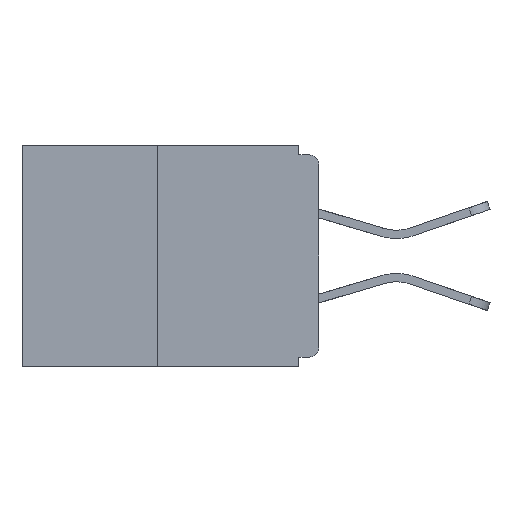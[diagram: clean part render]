
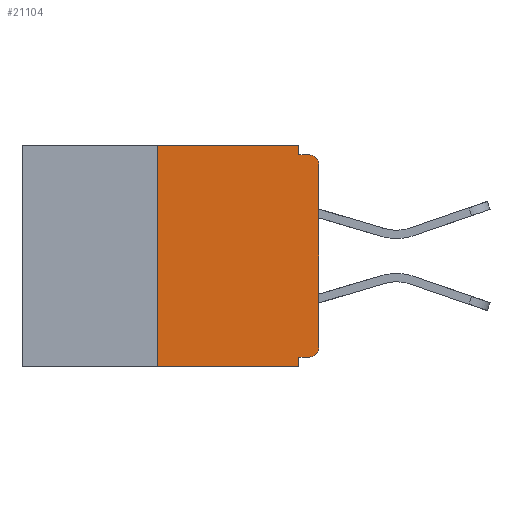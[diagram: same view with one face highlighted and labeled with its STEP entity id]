
A CAD part, left-side view. The second image highlights one B-rep face of the part: STEP entity #21104.
In plain terms, the highlighted planar face has unit normal (-1, 0, 0).
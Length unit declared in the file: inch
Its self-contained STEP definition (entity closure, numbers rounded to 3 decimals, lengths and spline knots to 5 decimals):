
#476 = DIRECTION ( 'NONE',  ( 0., 0., 1. ) ) ;
#1925 = ORIENTED_EDGE ( 'NONE', *, *, #23417, .F. ) ;
#2203 = VERTEX_POINT ( 'NONE', #7121 ) ;
#2289 = EDGE_CURVE ( 'NONE', #20654, #20920, #18518, .T. ) ;
#2533 = CARTESIAN_POINT ( 'NONE',  ( 0., 0.46, 0. ) ) ;
#2601 = EDGE_LOOP ( 'NONE', ( #22878, #6799, #9695, #23954, #12392, #19267, #4826, #17020, #1925, #10896 ) ) ;
#2767 = PLANE ( 'NONE',  #15764 ) ;
#2770 = CARTESIAN_POINT ( 'NONE',  ( 0., 0.25, 0. ) ) ;
#3852 = EDGE_CURVE ( 'NONE', #21690, #20055, #19896, .T. ) ;
#4244 = CARTESIAN_POINT ( 'NONE',  ( 0., 0.46, 0. ) ) ;
#4379 = VERTEX_POINT ( 'NONE', #20947 ) ;
#4826 = ORIENTED_EDGE ( 'NONE', *, *, #19658, .T. ) ;
#5192 = FACE_OUTER_BOUND ( 'NONE', #2601, .T. ) ;
#5286 = EDGE_CURVE ( 'NONE', #2203, #10711, #18366, .T. ) ;
#5598 = VERTEX_POINT ( 'NONE', #2770 ) ;
#5928 = VECTOR ( 'NONE', #20746, 39.37008 ) ;
#5968 = LINE ( 'NONE', #9209, #15302 ) ;
#6614 = VECTOR ( 'NONE', #17550, 39.37008 ) ;
#6799 = ORIENTED_EDGE ( 'NONE', *, *, #11990, .F. ) ;
#6907 = DIRECTION ( 'NONE',  ( 0., 0., -1. ) ) ;
#7121 = CARTESIAN_POINT ( 'NONE',  ( 0., 0.015, -0.328 ) ) ;
#7600 = DIRECTION ( 'NONE',  ( 0., 0., 1. ) ) ;
#7608 = DIRECTION ( 'NONE',  ( 0., 0., -1. ) ) ;
#7789 = EDGE_CURVE ( 'NONE', #2203, #23434, #19335, .T. ) ;
#7893 = VECTOR ( 'NONE', #19239, 39.37008 ) ;
#8104 = LINE ( 'NONE', #13598, #12831 ) ;
#9209 = CARTESIAN_POINT ( 'NONE',  ( 0., 0.031, 0. ) ) ;
#9425 = CARTESIAN_POINT ( 'NONE',  ( 0., 0., -0.015 ) ) ;
#9695 = ORIENTED_EDGE ( 'NONE', *, *, #3852, .T. ) ;
#9781 = VECTOR ( 'NONE', #24163, 39.37008 ) ;
#10086 = DIRECTION ( 'NONE',  ( 1., 0., 0. ) ) ;
#10711 = VERTEX_POINT ( 'NONE', #21001 ) ;
#10741 = EDGE_CURVE ( 'NONE', #5598, #19440, #15689, .T. ) ;
#10896 = ORIENTED_EDGE ( 'NONE', *, *, #11846, .F. ) ;
#11138 = CARTESIAN_POINT ( 'NONE',  ( 0., 0.031, 0. ) ) ;
#11846 = EDGE_CURVE ( 'NONE', #19440, #4379, #5968, .T. ) ;
#11990 = EDGE_CURVE ( 'NONE', #21690, #5598, #22936, .T. ) ;
#12392 = ORIENTED_EDGE ( 'NONE', *, *, #7789, .F. ) ;
#12660 = CARTESIAN_POINT ( 'NONE',  ( 0., 0., -0.03 ) ) ;
#12831 = VECTOR ( 'NONE', #476, 39.37008 ) ;
#13597 = LINE ( 'NONE', #14649, #9781 ) ;
#13598 = CARTESIAN_POINT ( 'NONE',  ( 0., 0., 0. ) ) ;
#14649 = CARTESIAN_POINT ( 'NONE',  ( 0., 0.031, -0.343 ) ) ;
#14977 = CARTESIAN_POINT ( 'NONE',  ( 0., 0.031, -0.328 ) ) ;
#15013 = CARTESIAN_POINT ( 'NONE',  ( 0., 0.25, 0. ) ) ;
#15017 = DIRECTION ( 'NONE',  ( -1., 0., 0. ) ) ;
#15302 = VECTOR ( 'NONE', #16848, 39.37008 ) ;
#15539 = CARTESIAN_POINT ( 'NONE',  ( 0., 0.46, -0.343 ) ) ;
#15664 = AXIS2_PLACEMENT_3D ( 'NONE', #17167, #15017, #7608 ) ;
#15689 = LINE ( 'NONE', #4244, #6614 ) ;
#15764 = AXIS2_PLACEMENT_3D ( 'NONE', #2533, #10086, #23194 ) ;
#16848 = DIRECTION ( 'NONE',  ( 0., 0., -1. ) ) ;
#17020 = ORIENTED_EDGE ( 'NONE', *, *, #2289, .T. ) ;
#17054 = LINE ( 'NONE', #9425, #5928 ) ;
#17167 = CARTESIAN_POINT ( 'NONE',  ( 0., 0.015, -0.03 ) ) ;
#17550 = DIRECTION ( 'NONE',  ( 0., -1., 0. ) ) ;
#17764 = CARTESIAN_POINT ( 'NONE',  ( 0., 0.25, -0.343 ) ) ;
#17944 = CARTESIAN_POINT ( 'NONE',  ( 0., 0.015, -0.313 ) ) ;
#17952 = VECTOR ( 'NONE', #7600, 39.37008 ) ;
#18366 = CIRCLE ( 'NONE', #20612, 0.015 ) ;
#18442 = VECTOR ( 'NONE', #23558, 39.37008 ) ;
#18518 = CIRCLE ( 'NONE', #15664, 0.015 ) ;
#19239 = DIRECTION ( 'NONE',  ( 0., -1., 0. ) ) ;
#19267 = ORIENTED_EDGE ( 'NONE', *, *, #5286, .T. ) ;
#19335 = LINE ( 'NONE', #21671, #18442 ) ;
#19440 = VERTEX_POINT ( 'NONE', #11138 ) ;
#19658 = EDGE_CURVE ( 'NONE', #10711, #20654, #8104, .T. ) ;
#19896 = LINE ( 'NONE', #15539, #7893 ) ;
#19999 = DIRECTION ( 'NONE',  ( -1., 0., 0. ) ) ;
#20055 = VERTEX_POINT ( 'NONE', #20285 ) ;
#20285 = CARTESIAN_POINT ( 'NONE',  ( 0., 0.031, -0.343 ) ) ;
#20612 = AXIS2_PLACEMENT_3D ( 'NONE', #17944, #19999, #6907 ) ;
#20654 = VERTEX_POINT ( 'NONE', #12660 ) ;
#20746 = DIRECTION ( 'NONE',  ( 0., -1., 0. ) ) ;
#20920 = VERTEX_POINT ( 'NONE', #22708 ) ;
#20947 = CARTESIAN_POINT ( 'NONE',  ( 0., 0.031, -0.015 ) ) ;
#21001 = CARTESIAN_POINT ( 'NONE',  ( 0., 0., -0.313 ) ) ;
#21104 = ADVANCED_FACE ( 'NONE', ( #5192 ), #2767, .F. ) ;
#21671 = CARTESIAN_POINT ( 'NONE',  ( 0., 0., -0.328 ) ) ;
#21690 = VERTEX_POINT ( 'NONE', #17764 ) ;
#22033 = EDGE_CURVE ( 'NONE', #23434, #20055, #13597, .T. ) ;
#22708 = CARTESIAN_POINT ( 'NONE',  ( 0., 0.015, -0.015 ) ) ;
#22878 = ORIENTED_EDGE ( 'NONE', *, *, #10741, .F. ) ;
#22936 = LINE ( 'NONE', #15013, #17952 ) ;
#23194 = DIRECTION ( 'NONE',  ( 0., 0., -1. ) ) ;
#23417 = EDGE_CURVE ( 'NONE', #4379, #20920, #17054, .T. ) ;
#23434 = VERTEX_POINT ( 'NONE', #14977 ) ;
#23558 = DIRECTION ( 'NONE',  ( 0., 1., 0. ) ) ;
#23954 = ORIENTED_EDGE ( 'NONE', *, *, #22033, .F. ) ;
#24163 = DIRECTION ( 'NONE',  ( 0., 0., -1. ) ) ;
